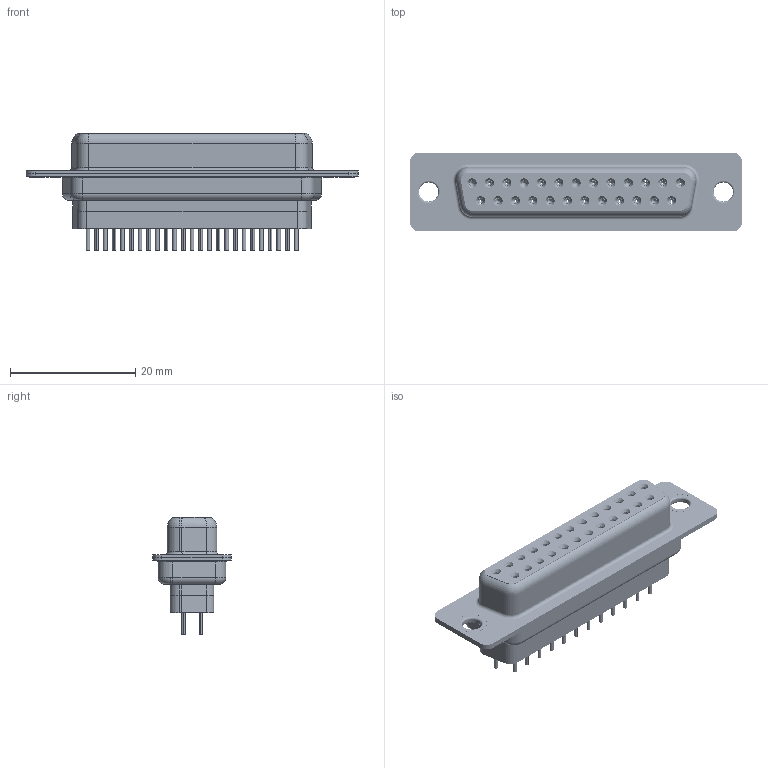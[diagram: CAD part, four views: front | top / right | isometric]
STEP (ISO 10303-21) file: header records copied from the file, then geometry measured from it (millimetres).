
FILE_DESCRIPTION (( 'STEP AP203' ), '1' );
FILE_NAME ('628-025-228-061.STEP', '2020-07-20T23:48:35', ( '' ), ( '' ), 'SwSTEP 2.0', 'SolidWorks 2020', '' );
FILE_SCHEMA (( 'CONFIG_CONTROL_DESIGN' ));
Length unit declared in the file: millimetre
Products named in the file (7): 628 Shell Rear_25 Contacts; 628 Contact Row 2_28L; 628 Housing_25 FF; 628 Shell Front_25 Contacts; 628 Thru Hole Rivet; 628-025-228-061; 628 Contact Row 1_28L
Assembly tree (30 placements, depth 2):
  628-025-228-061
    628 Housing_25 FF
    628 Shell Front_25 Contacts
    628 Shell Rear_25 Contacts
    628 Contact Row 1_28L  x13
    628 Contact Row 2_28L  x12
    628 Thru Hole Rivet  x2
Bounding box: 53 x 12.6 x 18.8 mm (x, y, z)
Volume: 4344.7 mm3; surface area: 10323.2 mm2
Topology: 31 solids, 31 shells, 3489 faces, 8880 edges, 5514 vertices
Faces by surface type: cylinder 1001, plane 848, torus 715, bspline 500, cone 425
Entity records: 28339 total; most frequent: CARTESIAN_POINT 6728, DIRECTION 4506, ORIENTED_EDGE 4044, EDGE_CURVE 2022, AXIS2_PLACEMENT_3D 1891, VERTEX_POINT 1277, CIRCLE 1055, EDGE_LOOP 1041
